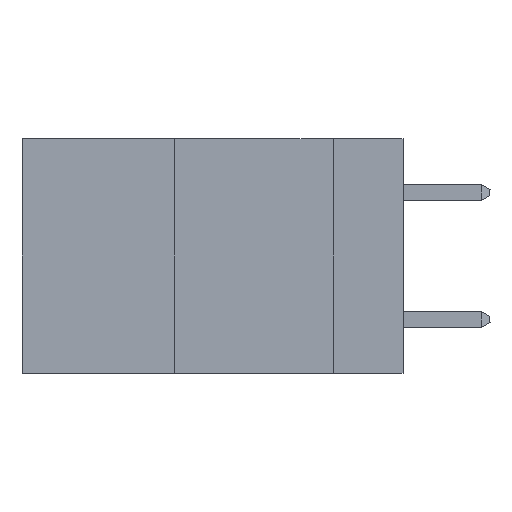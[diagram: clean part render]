
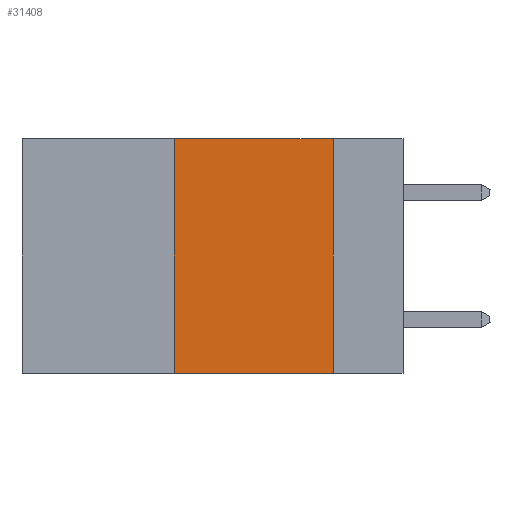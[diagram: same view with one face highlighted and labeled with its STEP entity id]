
A CAD part, left-side view. The second image highlights one B-rep face of the part: STEP entity #31408.
In plain terms, the highlighted planar face has unit normal (-1, 0, 0).
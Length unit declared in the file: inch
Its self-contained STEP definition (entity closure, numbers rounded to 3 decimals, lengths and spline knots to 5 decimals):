
#330 = FACE_OUTER_BOUND ( 'NONE', #20899, .T. ) ;
#2395 = CARTESIAN_POINT ( 'NONE',  ( 0., 0.11, -0.37 ) ) ;
#4352 = VECTOR ( 'NONE', #34100, 39.37008 ) ;
#5920 = EDGE_CURVE ( 'NONE', #19993, #20452, #37913, .T. ) ;
#8696 = VERTEX_POINT ( 'NONE', #2395 ) ;
#8770 = VERTEX_POINT ( 'NONE', #28367 ) ;
#8987 = DIRECTION ( 'NONE',  ( 0., 0., -1. ) ) ;
#9438 = LINE ( 'NONE', #31016, #38254 ) ;
#12162 = CARTESIAN_POINT ( 'NONE',  ( 0., 0.36, 0. ) ) ;
#14107 = DIRECTION ( 'NONE',  ( 0., 0., -1. ) ) ;
#16324 = ORIENTED_EDGE ( 'NONE', *, *, #35210, .F. ) ;
#17608 = CARTESIAN_POINT ( 'NONE',  ( 0., 0.36, -0.37 ) ) ;
#18057 = PLANE ( 'NONE',  #34583 ) ;
#18390 = CARTESIAN_POINT ( 'NONE',  ( 0., 0.6, -0.37 ) ) ;
#19993 = VERTEX_POINT ( 'NONE', #17608 ) ;
#20452 = VERTEX_POINT ( 'NONE', #20836 ) ;
#20836 = CARTESIAN_POINT ( 'NONE',  ( 0., 0.36, 0. ) ) ;
#20899 = EDGE_LOOP ( 'NONE', ( #16324, #30921, #21424, #32642 ) ) ;
#21424 = ORIENTED_EDGE ( 'NONE', *, *, #5920, .F. ) ;
#23178 = LINE ( 'NONE', #18390, #4352 ) ;
#23801 = VECTOR ( 'NONE', #24263, 39.37008 ) ;
#24263 = DIRECTION ( 'NONE',  ( 0., -1., 0. ) ) ;
#24452 = DIRECTION ( 'NONE',  ( 0., 0., 1. ) ) ;
#24953 = LINE ( 'NONE', #39528, #23801 ) ;
#26727 = VECTOR ( 'NONE', #24452, 39.37008 ) ;
#28367 = CARTESIAN_POINT ( 'NONE',  ( 0., 0.11, 0. ) ) ;
#30921 = ORIENTED_EDGE ( 'NONE', *, *, #44311, .F. ) ;
#31016 = CARTESIAN_POINT ( 'NONE',  ( 0., 0.11, 0. ) ) ;
#31408 = ADVANCED_FACE ( 'NONE', ( #330 ), #18057, .F. ) ;
#32642 = ORIENTED_EDGE ( 'NONE', *, *, #32764, .T. ) ;
#32764 = EDGE_CURVE ( 'NONE', #19993, #8696, #23178, .T. ) ;
#32802 = CARTESIAN_POINT ( 'NONE',  ( 0., 0.6, 0. ) ) ;
#34100 = DIRECTION ( 'NONE',  ( 0., -1., 0. ) ) ;
#34583 = AXIS2_PLACEMENT_3D ( 'NONE', #32802, #36419, #14107 ) ;
#35210 = EDGE_CURVE ( 'NONE', #8770, #8696, #9438, .T. ) ;
#36419 = DIRECTION ( 'NONE',  ( 1., 0., 0. ) ) ;
#37913 = LINE ( 'NONE', #12162, #26727 ) ;
#38254 = VECTOR ( 'NONE', #8987, 39.37008 ) ;
#39528 = CARTESIAN_POINT ( 'NONE',  ( 0., 0.6, 0. ) ) ;
#44311 = EDGE_CURVE ( 'NONE', #20452, #8770, #24953, .T. ) ;
